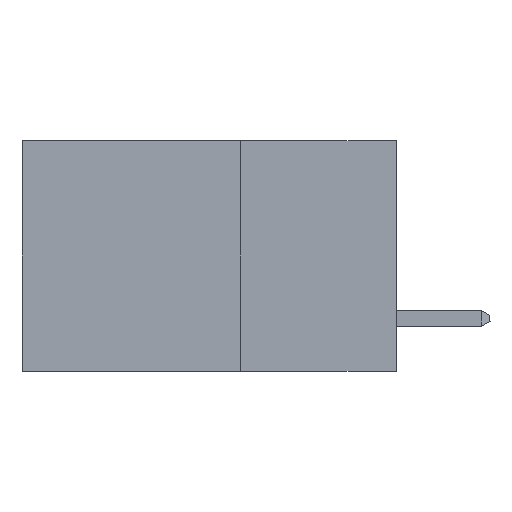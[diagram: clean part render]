
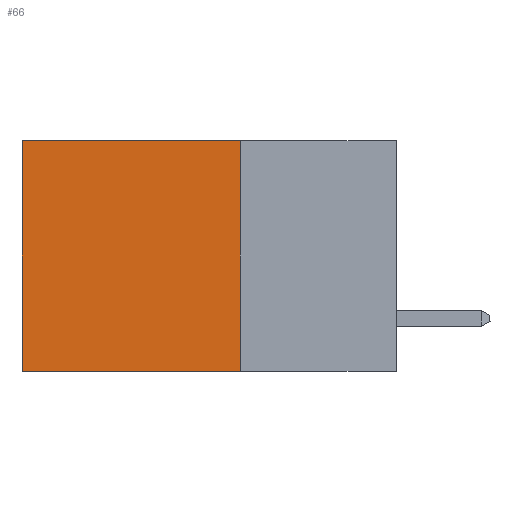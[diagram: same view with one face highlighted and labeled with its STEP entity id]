
A CAD part, left-side view. The second image highlights one B-rep face of the part: STEP entity #66.
In plain terms, the highlighted planar face has unit normal (-1, 0, 0).
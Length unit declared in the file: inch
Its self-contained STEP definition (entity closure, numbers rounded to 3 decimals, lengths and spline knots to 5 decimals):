
#66 = ADVANCED_FACE ( 'NONE', ( #5240 ), #9239, .F. ) ;
#96 = EDGE_CURVE ( 'NONE', #595, #4257, #8546, .T. ) ;
#530 = CARTESIAN_POINT ( 'NONE',  ( 0.298, 0.6, 0. ) ) ;
#595 = VERTEX_POINT ( 'NONE', #4657 ) ;
#849 = DIRECTION ( 'NONE',  ( 0., 0., -1. ) ) ;
#885 = VECTOR ( 'NONE', #7047, 39.37008 ) ;
#2806 = ORIENTED_EDGE ( 'NONE', *, *, #9170, .F. ) ;
#3015 = CARTESIAN_POINT ( 'NONE',  ( 0.298, 0.25, 0. ) ) ;
#3048 = DIRECTION ( 'NONE',  ( 0., 1., 0. ) ) ;
#3114 = CARTESIAN_POINT ( 'NONE',  ( 0.298, 0.25, 0. ) ) ;
#4110 = ORIENTED_EDGE ( 'NONE', *, *, #4950, .T. ) ;
#4257 = VERTEX_POINT ( 'NONE', #5890 ) ;
#4367 = CARTESIAN_POINT ( 'NONE',  ( 0.298, 0.25, 0. ) ) ;
#4657 = CARTESIAN_POINT ( 'NONE',  ( 0.298, 0.6, 0. ) ) ;
#4950 = EDGE_CURVE ( 'NONE', #9998, #595, #6130, .T. ) ;
#5240 = FACE_OUTER_BOUND ( 'NONE', #5407, .T. ) ;
#5305 = CARTESIAN_POINT ( 'NONE',  ( 0.298, 0.25, 0. ) ) ;
#5326 = ORIENTED_EDGE ( 'NONE', *, *, #96, .T. ) ;
#5407 = EDGE_LOOP ( 'NONE', ( #5326, #2806, #8166, #4110 ) ) ;
#5416 = VECTOR ( 'NONE', #8445, 39.37008 ) ;
#5447 = EDGE_CURVE ( 'NONE', #9998, #6101, #9041, .T. ) ;
#5890 = CARTESIAN_POINT ( 'NONE',  ( 0.298, 0.6, -0.37 ) ) ;
#6101 = VERTEX_POINT ( 'NONE', #9589 ) ;
#6130 = LINE ( 'NONE', #3015, #10162 ) ;
#6263 = VECTOR ( 'NONE', #849, 39.37008 ) ;
#6443 = AXIS2_PLACEMENT_3D ( 'NONE', #4367, #7672, #6787 ) ;
#6677 = LINE ( 'NONE', #6920, #5416 ) ;
#6787 = DIRECTION ( 'NONE',  ( 0., 0., -1. ) ) ;
#6920 = CARTESIAN_POINT ( 'NONE',  ( 0.298, 0.25, -0.37 ) ) ;
#7047 = DIRECTION ( 'NONE',  ( 0., 0., -1. ) ) ;
#7672 = DIRECTION ( 'NONE',  ( 1., 0., 0. ) ) ;
#8166 = ORIENTED_EDGE ( 'NONE', *, *, #5447, .F. ) ;
#8445 = DIRECTION ( 'NONE',  ( 0., 1., 0. ) ) ;
#8546 = LINE ( 'NONE', #530, #885 ) ;
#9041 = LINE ( 'NONE', #3114, #6263 ) ;
#9170 = EDGE_CURVE ( 'NONE', #6101, #4257, #6677, .T. ) ;
#9239 = PLANE ( 'NONE',  #6443 ) ;
#9589 = CARTESIAN_POINT ( 'NONE',  ( 0.298, 0.25, -0.37 ) ) ;
#9998 = VERTEX_POINT ( 'NONE', #5305 ) ;
#10162 = VECTOR ( 'NONE', #3048, 39.37008 ) ;
